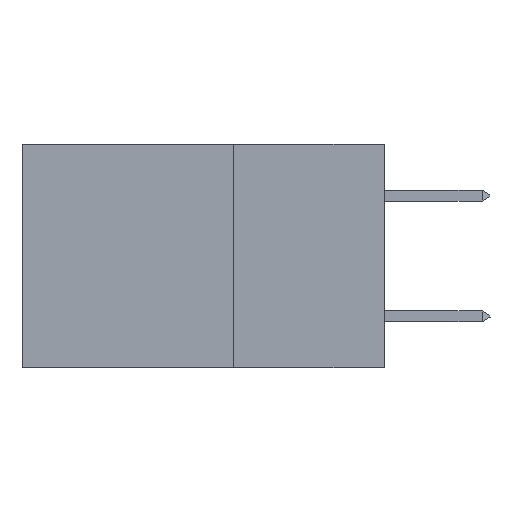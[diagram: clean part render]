
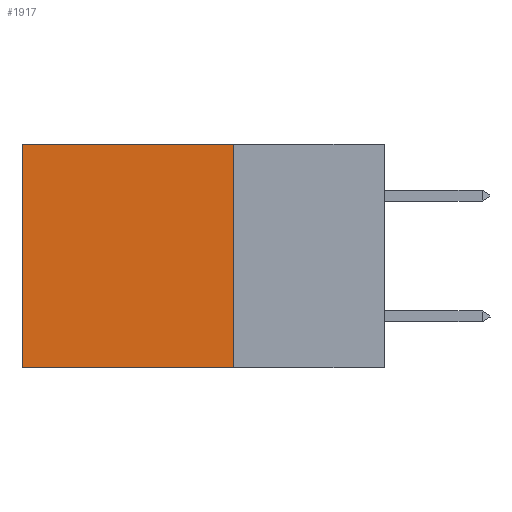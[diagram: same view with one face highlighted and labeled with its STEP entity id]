
A CAD part, left-side view. The second image highlights one B-rep face of the part: STEP entity #1917.
In plain terms, the highlighted planar face has unit normal (-1, 0, 0).
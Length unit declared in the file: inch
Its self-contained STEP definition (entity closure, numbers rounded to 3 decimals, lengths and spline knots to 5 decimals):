
#338 = EDGE_CURVE ( 'NONE', #13057, #10845, #5749, .T. ) ;
#502 = DIRECTION ( 'NONE',  ( 0., 0., -1. ) ) ;
#1917 = ADVANCED_FACE ( 'NONE', ( #3041 ), #3627, .F. ) ;
#2636 = CARTESIAN_POINT ( 'NONE',  ( 0.2875, 0.25, -0.37 ) ) ;
#3041 = FACE_OUTER_BOUND ( 'NONE', #17061, .T. ) ;
#3627 = PLANE ( 'NONE',  #5836 ) ;
#4763 = ORIENTED_EDGE ( 'NONE', *, *, #17143, .T. ) ;
#4935 = LINE ( 'NONE', #6431, #5478 ) ;
#5136 = DIRECTION ( 'NONE',  ( 0., 1., 0. ) ) ;
#5187 = VECTOR ( 'NONE', #13290, 39.37008 ) ;
#5291 = CARTESIAN_POINT ( 'NONE',  ( 0.2875, 0.25, -0.37 ) ) ;
#5478 = VECTOR ( 'NONE', #5136, 39.37008 ) ;
#5749 = LINE ( 'NONE', #15001, #10878 ) ;
#5795 = CARTESIAN_POINT ( 'NONE',  ( 0.2875, 0.25, 0. ) ) ;
#5836 = AXIS2_PLACEMENT_3D ( 'NONE', #6070, #15327, #9167 ) ;
#6070 = CARTESIAN_POINT ( 'NONE',  ( 0.2875, 0.25, 0. ) ) ;
#6431 = CARTESIAN_POINT ( 'NONE',  ( 0.2875, 0.25, 0. ) ) ;
#6624 = CARTESIAN_POINT ( 'NONE',  ( 0.2875, 0.6, 0. ) ) ;
#8546 = LINE ( 'NONE', #2636, #5187 ) ;
#9167 = DIRECTION ( 'NONE',  ( 0., 0., -1. ) ) ;
#10140 = ORIENTED_EDGE ( 'NONE', *, *, #18849, .F. ) ;
#10317 = ORIENTED_EDGE ( 'NONE', *, *, #15545, .T. ) ;
#10845 = VERTEX_POINT ( 'NONE', #5291 ) ;
#10878 = VECTOR ( 'NONE', #12260, 39.37008 ) ;
#11175 = VECTOR ( 'NONE', #502, 39.37008 ) ;
#11836 = ORIENTED_EDGE ( 'NONE', *, *, #338, .F. ) ;
#12260 = DIRECTION ( 'NONE',  ( 0., 0., -1. ) ) ;
#12522 = VERTEX_POINT ( 'NONE', #12674 ) ;
#12674 = CARTESIAN_POINT ( 'NONE',  ( 0.2875, 0.6, -0.37 ) ) ;
#13057 = VERTEX_POINT ( 'NONE', #5795 ) ;
#13290 = DIRECTION ( 'NONE',  ( 0., 1., 0. ) ) ;
#14680 = LINE ( 'NONE', #6624, #11175 ) ;
#15001 = CARTESIAN_POINT ( 'NONE',  ( 0.2875, 0.25, 0. ) ) ;
#15327 = DIRECTION ( 'NONE',  ( 1., 0., 0. ) ) ;
#15545 = EDGE_CURVE ( 'NONE', #16043, #12522, #14680, .T. ) ;
#16043 = VERTEX_POINT ( 'NONE', #17287 ) ;
#17061 = EDGE_LOOP ( 'NONE', ( #10317, #10140, #11836, #4763 ) ) ;
#17143 = EDGE_CURVE ( 'NONE', #13057, #16043, #4935, .T. ) ;
#17287 = CARTESIAN_POINT ( 'NONE',  ( 0.2875, 0.6, 0. ) ) ;
#18849 = EDGE_CURVE ( 'NONE', #10845, #12522, #8546, .T. ) ;
